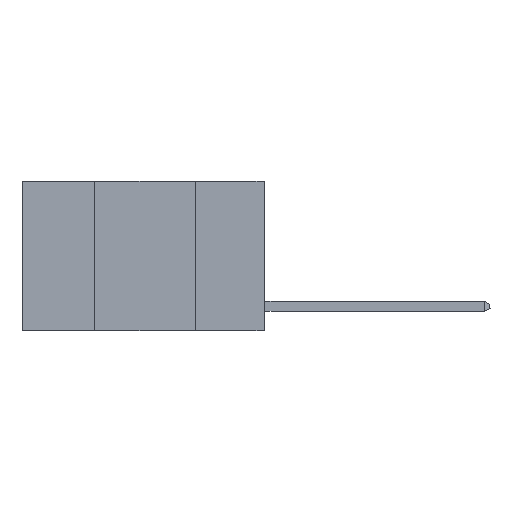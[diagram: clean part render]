
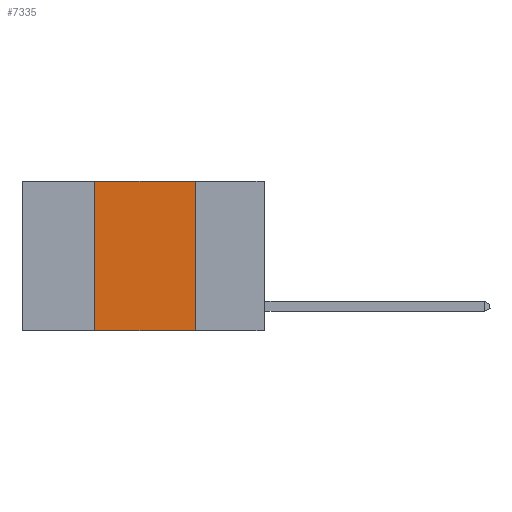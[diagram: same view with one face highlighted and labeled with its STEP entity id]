
A CAD part, left-side view. The second image highlights one B-rep face of the part: STEP entity #7335.
In plain terms, the highlighted planar face has unit normal (-1, 0, 0).
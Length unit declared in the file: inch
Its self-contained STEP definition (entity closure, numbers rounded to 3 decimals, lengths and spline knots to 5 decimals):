
#8 = DIRECTION ( 'NONE',  ( 0., 0., 1. ) ) ;
#117 = AXIS2_PLACEMENT_3D ( 'NONE', #6427, #6472, #7994 ) ;
#188 = CARTESIAN_POINT ( 'NONE',  ( 0., 0.42, -0.37 ) ) ;
#558 = CARTESIAN_POINT ( 'NONE',  ( 0., 0.6, -0.37 ) ) ;
#839 = CARTESIAN_POINT ( 'NONE',  ( 0., 0.17, 0. ) ) ;
#1656 = ORIENTED_EDGE ( 'NONE', *, *, #1810, .F. ) ;
#1810 = EDGE_CURVE ( 'NONE', #3489, #1826, #6637, .T. ) ;
#1826 = VERTEX_POINT ( 'NONE', #6931 ) ;
#1848 = VECTOR ( 'NONE', #6241, 39.37008 ) ;
#1880 = ORIENTED_EDGE ( 'NONE', *, *, #5664, .F. ) ;
#3403 = VECTOR ( 'NONE', #6514, 39.37008 ) ;
#3489 = VERTEX_POINT ( 'NONE', #4614 ) ;
#3744 = CARTESIAN_POINT ( 'NONE',  ( 0., 0.6, 0. ) ) ;
#3873 = EDGE_LOOP ( 'NONE', ( #5291, #1656, #1880, #5815 ) ) ;
#4200 = EDGE_CURVE ( 'NONE', #1826, #6625, #6917, .T. ) ;
#4216 = FACE_OUTER_BOUND ( 'NONE', #3873, .T. ) ;
#4614 = CARTESIAN_POINT ( 'NONE',  ( 0., 0.42, 0. ) ) ;
#5065 = EDGE_CURVE ( 'NONE', #5799, #6625, #5091, .T. ) ;
#5091 = LINE ( 'NONE', #558, #3403 ) ;
#5291 = ORIENTED_EDGE ( 'NONE', *, *, #4200, .F. ) ;
#5642 = PLANE ( 'NONE',  #117 ) ;
#5664 = EDGE_CURVE ( 'NONE', #5799, #3489, #9026, .T. ) ;
#5703 = VECTOR ( 'NONE', #6217, 39.37008 ) ;
#5799 = VERTEX_POINT ( 'NONE', #188 ) ;
#5815 = ORIENTED_EDGE ( 'NONE', *, *, #5065, .T. ) ;
#6217 = DIRECTION ( 'NONE',  ( 0., 0., -1. ) ) ;
#6241 = DIRECTION ( 'NONE',  ( 0., -1., 0. ) ) ;
#6427 = CARTESIAN_POINT ( 'NONE',  ( 0., 0.6, 0. ) ) ;
#6458 = CARTESIAN_POINT ( 'NONE',  ( 0., 0.17, -0.37 ) ) ;
#6472 = DIRECTION ( 'NONE',  ( 1., 0., 0. ) ) ;
#6514 = DIRECTION ( 'NONE',  ( 0., -1., 0. ) ) ;
#6625 = VERTEX_POINT ( 'NONE', #6458 ) ;
#6637 = LINE ( 'NONE', #3744, #1848 ) ;
#6917 = LINE ( 'NONE', #839, #5703 ) ;
#6931 = CARTESIAN_POINT ( 'NONE',  ( 0., 0.17, 0. ) ) ;
#7335 = ADVANCED_FACE ( 'NONE', ( #4216 ), #5642, .F. ) ;
#7994 = DIRECTION ( 'NONE',  ( 0., 0., -1. ) ) ;
#8982 = VECTOR ( 'NONE', #8, 39.37008 ) ;
#9026 = LINE ( 'NONE', #9611, #8982 ) ;
#9611 = CARTESIAN_POINT ( 'NONE',  ( 0., 0.42, 0. ) ) ;
